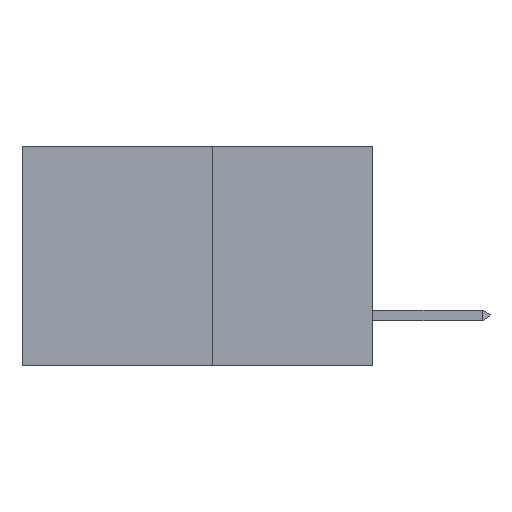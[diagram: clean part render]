
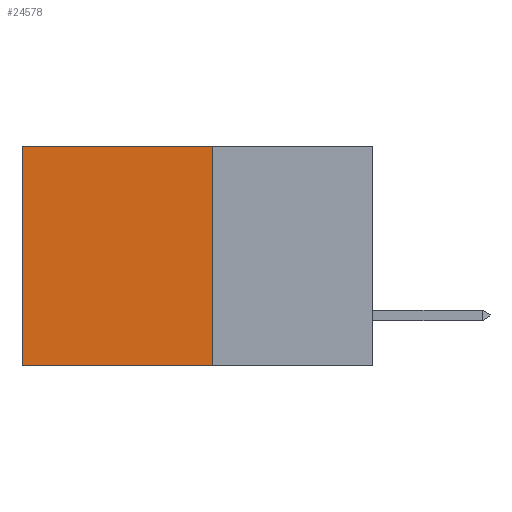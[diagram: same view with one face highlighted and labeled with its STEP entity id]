
A CAD part, left-side view. The second image highlights one B-rep face of the part: STEP entity #24578.
In plain terms, the highlighted planar face has unit normal (-1, 0, 0).
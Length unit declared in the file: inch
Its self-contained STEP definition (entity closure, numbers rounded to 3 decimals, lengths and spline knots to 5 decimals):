
#137 = CARTESIAN_POINT ( 'NONE',  ( 0.277, 0.59, -0.37 ) ) ;
#790 = CARTESIAN_POINT ( 'NONE',  ( 0.277, 0.27, -0.37 ) ) ;
#1998 = EDGE_CURVE ( 'NONE', #10715, #11352, #12470, .T. ) ;
#2105 = VECTOR ( 'NONE', #9849, 39.37008 ) ;
#2528 = DIRECTION ( 'NONE',  ( 0., 1., 0. ) ) ;
#2540 = EDGE_CURVE ( 'NONE', #20692, #11352, #13989, .T. ) ;
#2601 = ORIENTED_EDGE ( 'NONE', *, *, #2540, .T. ) ;
#2834 = DIRECTION ( 'NONE',  ( 0., 0., -1. ) ) ;
#3633 = VECTOR ( 'NONE', #12585, 39.37008 ) ;
#4151 = VERTEX_POINT ( 'NONE', #19641 ) ;
#5238 = FACE_OUTER_BOUND ( 'NONE', #23947, .T. ) ;
#7967 = ORIENTED_EDGE ( 'NONE', *, *, #16607, .T. ) ;
#9819 = CARTESIAN_POINT ( 'NONE',  ( 0.277, 0.27, -0.37 ) ) ;
#9823 = CARTESIAN_POINT ( 'NONE',  ( 0.277, 0.27, -0.37 ) ) ;
#9849 = DIRECTION ( 'NONE',  ( 0., 1., 0. ) ) ;
#10144 = CARTESIAN_POINT ( 'NONE',  ( 0.277, 0.59, 0. ) ) ;
#10715 = VERTEX_POINT ( 'NONE', #25418 ) ;
#11352 = VERTEX_POINT ( 'NONE', #13844 ) ;
#11770 = DIRECTION ( 'NONE',  ( 0., 0., -1. ) ) ;
#12470 = LINE ( 'NONE', #9819, #2105 ) ;
#12519 = PLANE ( 'NONE',  #22287 ) ;
#12585 = DIRECTION ( 'NONE',  ( 0., 0., -1. ) ) ;
#13023 = ORIENTED_EDGE ( 'NONE', *, *, #19317, .F. ) ;
#13844 = CARTESIAN_POINT ( 'NONE',  ( 0.277, 0.59, -0.37 ) ) ;
#13989 = LINE ( 'NONE', #137, #3633 ) ;
#14508 = DIRECTION ( 'NONE',  ( 1., 0., 0. ) ) ;
#15467 = ORIENTED_EDGE ( 'NONE', *, *, #1998, .F. ) ;
#16607 = EDGE_CURVE ( 'NONE', #4151, #20692, #23206, .T. ) ;
#17999 = VECTOR ( 'NONE', #2528, 39.37008 ) ;
#19317 = EDGE_CURVE ( 'NONE', #4151, #10715, #20207, .T. ) ;
#19641 = CARTESIAN_POINT ( 'NONE',  ( 0.277, 0.27, 0. ) ) ;
#20207 = LINE ( 'NONE', #9823, #24795 ) ;
#20692 = VERTEX_POINT ( 'NONE', #10144 ) ;
#22287 = AXIS2_PLACEMENT_3D ( 'NONE', #790, #14508, #2834 ) ;
#23206 = LINE ( 'NONE', #23989, #17999 ) ;
#23947 = EDGE_LOOP ( 'NONE', ( #2601, #15467, #13023, #7967 ) ) ;
#23989 = CARTESIAN_POINT ( 'NONE',  ( 0.277, 0.27, 0. ) ) ;
#24578 = ADVANCED_FACE ( 'NONE', ( #5238 ), #12519, .F. ) ;
#24795 = VECTOR ( 'NONE', #11770, 39.37008 ) ;
#25418 = CARTESIAN_POINT ( 'NONE',  ( 0.277, 0.27, -0.37 ) ) ;
